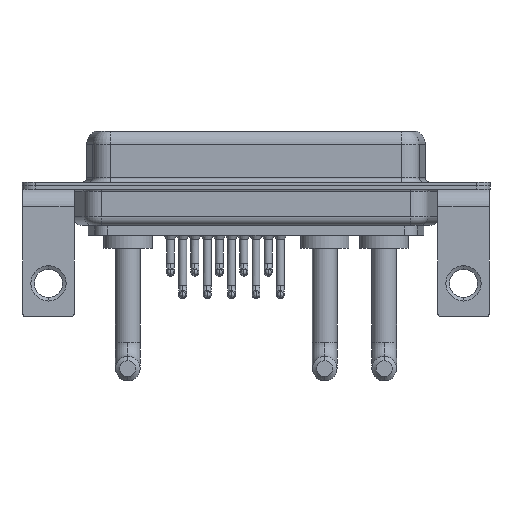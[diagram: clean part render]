
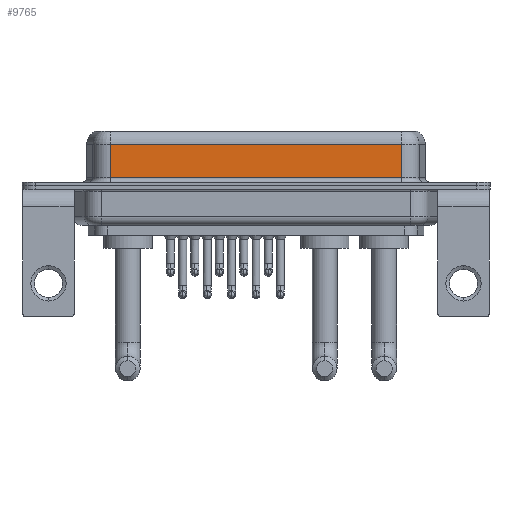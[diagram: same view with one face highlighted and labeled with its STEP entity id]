
A CAD part, front view. The second image highlights one B-rep face of the part: STEP entity #9765.
In plain terms, the highlighted planar face has unit normal (0, -1, 0).
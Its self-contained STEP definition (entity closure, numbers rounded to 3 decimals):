
#34 = ORIENTED_EDGE ( 'NONE', *, *, #3048, .F. ) ;
#525 = CARTESIAN_POINT ( 'NONE',  ( 40.037, -3.95, 4.65 ) ) ;
#1139 = EDGE_CURVE ( 'NONE', #13051, #19644, #11784, .T. ) ;
#1254 = CARTESIAN_POINT ( 'NONE',  ( 7.013, -3.95, 0.9 ) ) ;
#2137 = DIRECTION ( 'NONE',  ( 1., 0., 0. ) ) ;
#3008 = FACE_OUTER_BOUND ( 'NONE', #19569, .T. ) ;
#3048 = EDGE_CURVE ( 'NONE', #5029, #3640, #7748, .T. ) ;
#3640 = VERTEX_POINT ( 'NONE', #6652 ) ;
#5029 = VERTEX_POINT ( 'NONE', #10241 ) ;
#6536 = CARTESIAN_POINT ( 'NONE',  ( 7.013, -3.95, 4.65 ) ) ;
#6549 = CARTESIAN_POINT ( 'NONE',  ( 40.037, -3.95, 0.9 ) ) ;
#6652 = CARTESIAN_POINT ( 'NONE',  ( 40.037, -3.95, 0.9 ) ) ;
#7381 = CARTESIAN_POINT ( 'NONE',  ( 7.013, -3.95, 6.4 ) ) ;
#7519 = EDGE_CURVE ( 'NONE', #19644, #3640, #8245, .T. ) ;
#7606 = CARTESIAN_POINT ( 'NONE',  ( 40.037, -3.95, 6.4 ) ) ;
#7748 = LINE ( 'NONE', #18465, #18744 ) ;
#8044 = DIRECTION ( 'NONE',  ( 0., 0., -1. ) ) ;
#8245 = LINE ( 'NONE', #6549, #17140 ) ;
#9100 = DIRECTION ( 'NONE',  ( 0., 0., 1. ) ) ;
#9602 = ORIENTED_EDGE ( 'NONE', *, *, #7519, .T. ) ;
#9765 = ADVANCED_FACE ( 'NONE', ( #3008 ), #10312, .F. ) ;
#10241 = CARTESIAN_POINT ( 'NONE',  ( 40.037, -3.95, 4.65 ) ) ;
#10312 = PLANE ( 'NONE',  #19771 ) ;
#11784 = LINE ( 'NONE', #7381, #13083 ) ;
#12845 = DIRECTION ( 'NONE',  ( -1., 0., 0. ) ) ;
#13051 = VERTEX_POINT ( 'NONE', #6536 ) ;
#13083 = VECTOR ( 'NONE', #15181, 1000. ) ;
#13429 = ORIENTED_EDGE ( 'NONE', *, *, #1139, .T. ) ;
#13998 = DIRECTION ( 'NONE',  ( 0., 1., 0. ) ) ;
#14445 = LINE ( 'NONE', #525, #14519 ) ;
#14519 = VECTOR ( 'NONE', #12845, 1000. ) ;
#15181 = DIRECTION ( 'NONE',  ( 0., 0., -1. ) ) ;
#16425 = EDGE_CURVE ( 'NONE', #5029, #13051, #14445, .T. ) ;
#17140 = VECTOR ( 'NONE', #2137, 1000. ) ;
#18465 = CARTESIAN_POINT ( 'NONE',  ( 40.037, -3.95, 6.4 ) ) ;
#18744 = VECTOR ( 'NONE', #8044, 1000. ) ;
#19569 = EDGE_LOOP ( 'NONE', ( #34, #19777, #13429, #9602 ) ) ;
#19644 = VERTEX_POINT ( 'NONE', #1254 ) ;
#19771 = AXIS2_PLACEMENT_3D ( 'NONE', #7606, #13998, #9100 ) ;
#19777 = ORIENTED_EDGE ( 'NONE', *, *, #16425, .T. ) ;
